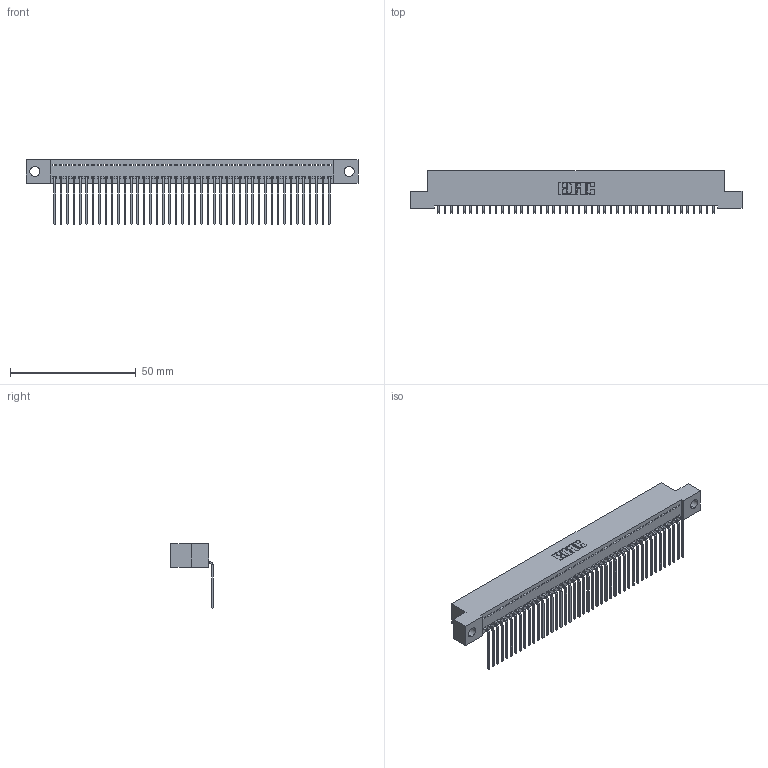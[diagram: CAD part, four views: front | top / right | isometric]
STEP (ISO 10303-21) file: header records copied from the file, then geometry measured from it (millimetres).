
FILE_DESCRIPTION (( 'STEP AP203' ), '1' );
FILE_NAME ('342-044-559-104.STEP', '2018-08-12T15:03:22', ( '' ), ( '' ), 'SwSTEP 2.0', 'SolidWorks 2016', '' );
FILE_SCHEMA (( 'CONFIG_CONTROL_DESIGN' ));
Length unit declared in the file: inch
Products named in the file (3): 342 Part_.156 TH; 345-292-001_558 559 Tail - 1; 342-044-559-104
Assembly tree (45 placements, depth 2):
  342-044-559-104
    342 Part_.156 TH
    345-292-001_558 559 Tail - 1  x44
Bounding box: 132.08 x 16.83 x 25.78 mm (x, y, z)
Volume: 11647.7 mm3; surface area: 17792.8 mm2
Topology: 45 solids, 45 shells, 2750 faces, 8307 edges, 5478 vertices
Faces by surface type: plane 2002, cylinder 748
Entity records: 26595 total; most frequent: CARTESIAN_POINT 4594, ORIENTED_EDGE 4574, DIRECTION 3871, EDGE_CURVE 2287, LINE 2159, VECTOR 2159, VERTEX_POINT 1522, AXIS2_PLACEMENT_3D 856
